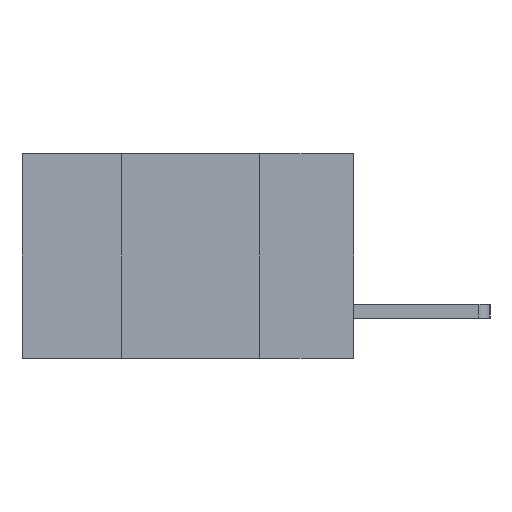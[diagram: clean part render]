
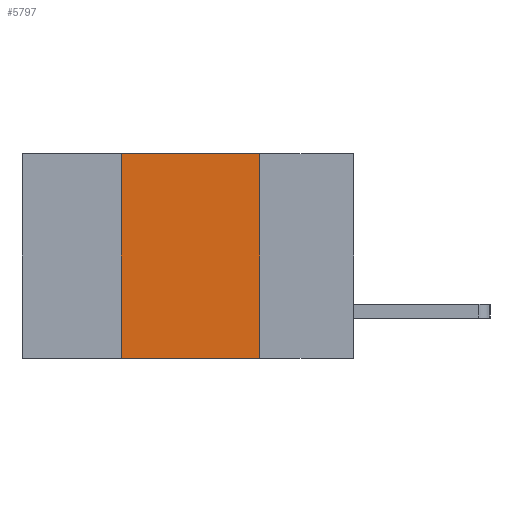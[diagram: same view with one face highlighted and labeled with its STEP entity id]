
A CAD part, left-side view. The second image highlights one B-rep face of the part: STEP entity #5797.
In plain terms, the highlighted planar face has unit normal (-1, 0, 0).
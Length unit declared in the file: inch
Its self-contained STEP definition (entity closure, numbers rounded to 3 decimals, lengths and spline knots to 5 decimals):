
#370 = CARTESIAN_POINT ( 'NONE',  ( 0., 0.17, 0. ) ) ;
#550 = CARTESIAN_POINT ( 'NONE',  ( 0., 0.17, 0. ) ) ;
#650 = ORIENTED_EDGE ( 'NONE', *, *, #1376, .F. ) ;
#764 = VERTEX_POINT ( 'NONE', #5520 ) ;
#1196 = VECTOR ( 'NONE', #7675, 39.37008 ) ;
#1376 = EDGE_CURVE ( 'NONE', #9536, #12355, #4116, .T. ) ;
#2309 = DIRECTION ( 'NONE',  ( 0., -1., 0. ) ) ;
#3236 = LINE ( 'NONE', #12603, #3439 ) ;
#3259 = EDGE_CURVE ( 'NONE', #13931, #9536, #10226, .T. ) ;
#3296 = CARTESIAN_POINT ( 'NONE',  ( 0., 0.6, -0.37 ) ) ;
#3332 = ORIENTED_EDGE ( 'NONE', *, *, #3259, .F. ) ;
#3439 = VECTOR ( 'NONE', #5596, 39.37008 ) ;
#3884 = PLANE ( 'NONE',  #11070 ) ;
#3959 = CARTESIAN_POINT ( 'NONE',  ( 0., 0.6, 0. ) ) ;
#4116 = LINE ( 'NONE', #550, #5386 ) ;
#4253 = CARTESIAN_POINT ( 'NONE',  ( 0., 0.17, -0.37 ) ) ;
#5386 = VECTOR ( 'NONE', #13182, 39.37008 ) ;
#5520 = CARTESIAN_POINT ( 'NONE',  ( 0., 0.42, -0.37 ) ) ;
#5596 = DIRECTION ( 'NONE',  ( 0., 0., 1. ) ) ;
#5797 = ADVANCED_FACE ( 'NONE', ( #12956 ), #3884, .F. ) ;
#5987 = ORIENTED_EDGE ( 'NONE', *, *, #6917, .F. ) ;
#6464 = CARTESIAN_POINT ( 'NONE',  ( 0., 0.6, 0. ) ) ;
#6917 = EDGE_CURVE ( 'NONE', #764, #13931, #3236, .T. ) ;
#7675 = DIRECTION ( 'NONE',  ( 0., -1., 0. ) ) ;
#9201 = LINE ( 'NONE', #3296, #11181 ) ;
#9536 = VERTEX_POINT ( 'NONE', #370 ) ;
#10226 = LINE ( 'NONE', #6464, #1196 ) ;
#10235 = EDGE_CURVE ( 'NONE', #764, #12355, #9201, .T. ) ;
#11038 = CARTESIAN_POINT ( 'NONE',  ( 0., 0.42, 0. ) ) ;
#11070 = AXIS2_PLACEMENT_3D ( 'NONE', #3959, #13175, #11979 ) ;
#11181 = VECTOR ( 'NONE', #2309, 39.37008 ) ;
#11367 = EDGE_LOOP ( 'NONE', ( #650, #3332, #5987, #11638 ) ) ;
#11638 = ORIENTED_EDGE ( 'NONE', *, *, #10235, .T. ) ;
#11979 = DIRECTION ( 'NONE',  ( 0., 0., -1. ) ) ;
#12355 = VERTEX_POINT ( 'NONE', #4253 ) ;
#12603 = CARTESIAN_POINT ( 'NONE',  ( 0., 0.42, 0. ) ) ;
#12956 = FACE_OUTER_BOUND ( 'NONE', #11367, .T. ) ;
#13175 = DIRECTION ( 'NONE',  ( 1., 0., 0. ) ) ;
#13182 = DIRECTION ( 'NONE',  ( 0., 0., -1. ) ) ;
#13931 = VERTEX_POINT ( 'NONE', #11038 ) ;
